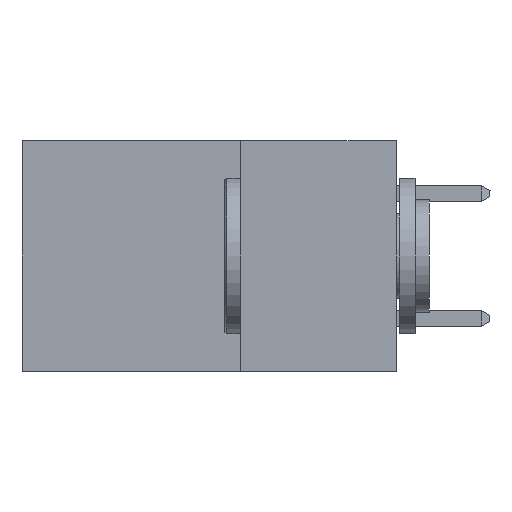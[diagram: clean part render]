
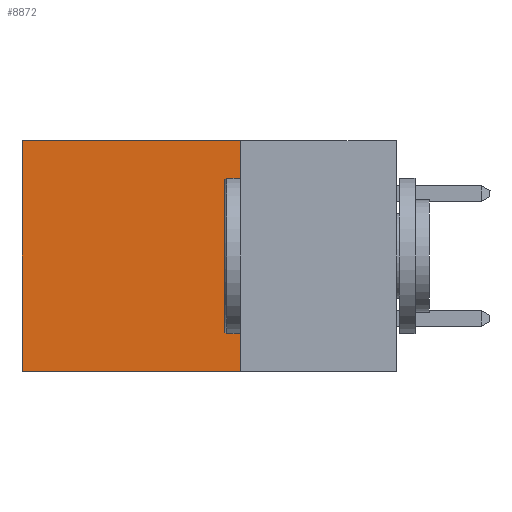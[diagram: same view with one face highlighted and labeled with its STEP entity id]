
A CAD part, left-side view. The second image highlights one B-rep face of the part: STEP entity #8872.
In plain terms, the highlighted planar face has unit normal (-1, 0, 0).
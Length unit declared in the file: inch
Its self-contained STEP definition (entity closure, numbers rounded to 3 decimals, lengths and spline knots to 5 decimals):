
#409 = FACE_OUTER_BOUND ( 'NONE', #12371, .T. ) ;
#904 = LINE ( 'NONE', #11826, #15070 ) ;
#1540 = DIRECTION ( 'NONE',  ( 0., 1., 0. ) ) ;
#1623 = VERTEX_POINT ( 'NONE', #16991 ) ;
#2036 = LINE ( 'NONE', #12028, #8892 ) ;
#2477 = CARTESIAN_POINT ( 'NONE',  ( 0.298, 0.25, 0. ) ) ;
#2927 = ORIENTED_EDGE ( 'NONE', *, *, #7743, .T. ) ;
#3052 = VECTOR ( 'NONE', #1540, 39.37008 ) ;
#3095 = LINE ( 'NONE', #17179, #9913 ) ;
#3773 = AXIS2_PLACEMENT_3D ( 'NONE', #2477, #8017, #17464 ) ;
#6495 = DIRECTION ( 'NONE',  ( 0., 1., 0. ) ) ;
#6558 = ORIENTED_EDGE ( 'NONE', *, *, #14638, .T. ) ;
#6735 = LINE ( 'NONE', #8416, #3052 ) ;
#7736 = DIRECTION ( 'NONE',  ( 0., 0., -1. ) ) ;
#7743 = EDGE_CURVE ( 'NONE', #1623, #15433, #2036, .T. ) ;
#7775 = ORIENTED_EDGE ( 'NONE', *, *, #11330, .F. ) ;
#8017 = DIRECTION ( 'NONE',  ( 1., 0., 0. ) ) ;
#8416 = CARTESIAN_POINT ( 'NONE',  ( 0.298, 0.25, 0. ) ) ;
#8699 = CARTESIAN_POINT ( 'NONE',  ( 0.298, 0.25, -0.37 ) ) ;
#8741 = EDGE_CURVE ( 'NONE', #13716, #13015, #3095, .T. ) ;
#8872 = ADVANCED_FACE ( 'NONE', ( #409 ), #16117, .F. ) ;
#8892 = VECTOR ( 'NONE', #11652, 39.37008 ) ;
#9913 = VECTOR ( 'NONE', #7736, 39.37008 ) ;
#10089 = CARTESIAN_POINT ( 'NONE',  ( 0.298, 0.25, 0. ) ) ;
#11330 = EDGE_CURVE ( 'NONE', #13015, #15433, #904, .T. ) ;
#11652 = DIRECTION ( 'NONE',  ( 0., 0., -1. ) ) ;
#11826 = CARTESIAN_POINT ( 'NONE',  ( 0.298, 0.25, -0.37 ) ) ;
#12028 = CARTESIAN_POINT ( 'NONE',  ( 0.298, 0.6, 0. ) ) ;
#12371 = EDGE_LOOP ( 'NONE', ( #2927, #7775, #17068, #6558 ) ) ;
#12762 = CARTESIAN_POINT ( 'NONE',  ( 0.298, 0.6, -0.37 ) ) ;
#13015 = VERTEX_POINT ( 'NONE', #8699 ) ;
#13716 = VERTEX_POINT ( 'NONE', #10089 ) ;
#14638 = EDGE_CURVE ( 'NONE', #13716, #1623, #6735, .T. ) ;
#15070 = VECTOR ( 'NONE', #6495, 39.37008 ) ;
#15433 = VERTEX_POINT ( 'NONE', #12762 ) ;
#16117 = PLANE ( 'NONE',  #3773 ) ;
#16991 = CARTESIAN_POINT ( 'NONE',  ( 0.298, 0.6, 0. ) ) ;
#17068 = ORIENTED_EDGE ( 'NONE', *, *, #8741, .F. ) ;
#17179 = CARTESIAN_POINT ( 'NONE',  ( 0.298, 0.25, 0. ) ) ;
#17464 = DIRECTION ( 'NONE',  ( 0., 0., -1. ) ) ;
